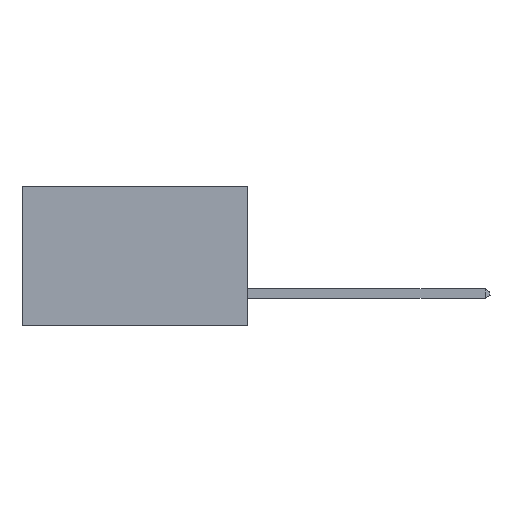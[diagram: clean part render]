
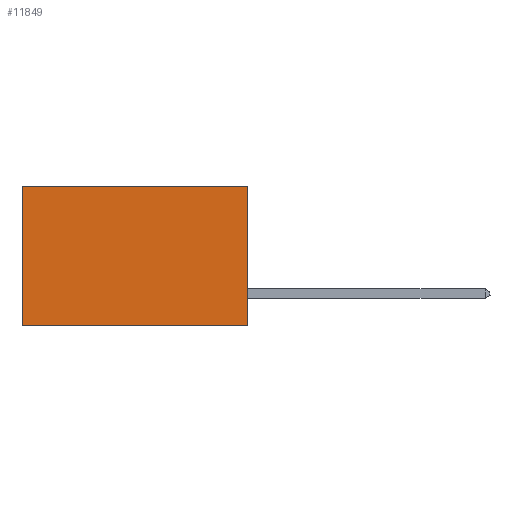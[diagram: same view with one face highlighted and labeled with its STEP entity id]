
A CAD part, left-side view. The second image highlights one B-rep face of the part: STEP entity #11849.
In plain terms, the highlighted planar face has unit normal (-1, 0, 0).
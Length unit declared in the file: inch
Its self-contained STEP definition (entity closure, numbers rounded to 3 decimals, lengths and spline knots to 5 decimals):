
#145 = EDGE_CURVE ( 'NONE', #5645, #9036, #12371, .T. ) ;
#515 = EDGE_CURVE ( 'NONE', #6734, #9036, #594, .T. ) ;
#594 = LINE ( 'NONE', #8430, #11598 ) ;
#1111 = EDGE_CURVE ( 'NONE', #6306, #6734, #10936, .T. ) ;
#1329 = DIRECTION ( 'NONE',  ( 0., 0., -1. ) ) ;
#1531 = AXIS2_PLACEMENT_3D ( 'NONE', #2247, #9335, #3285 ) ;
#1947 = CARTESIAN_POINT ( 'NONE',  ( 0.298, 0., 0. ) ) ;
#2247 = CARTESIAN_POINT ( 'NONE',  ( 0.298, 0., 0. ) ) ;
#3099 = CARTESIAN_POINT ( 'NONE',  ( 0.298, 0., 0. ) ) ;
#3152 = VECTOR ( 'NONE', #6441, 39.37008 ) ;
#3285 = DIRECTION ( 'NONE',  ( 0., 0., -1. ) ) ;
#3694 = ORIENTED_EDGE ( 'NONE', *, *, #1111, .T. ) ;
#4475 = DIRECTION ( 'NONE',  ( 0., 0., -1. ) ) ;
#4659 = LINE ( 'NONE', #9530, #10099 ) ;
#5645 = VERTEX_POINT ( 'NONE', #8923 ) ;
#5964 = VECTOR ( 'NONE', #10267, 39.37008 ) ;
#6306 = VERTEX_POINT ( 'NONE', #1947 ) ;
#6441 = DIRECTION ( 'NONE',  ( 0., 1., 0. ) ) ;
#6734 = VERTEX_POINT ( 'NONE', #7531 ) ;
#7344 = ORIENTED_EDGE ( 'NONE', *, *, #515, .T. ) ;
#7531 = CARTESIAN_POINT ( 'NONE',  ( 0.298, 0.6, 0. ) ) ;
#8396 = CARTESIAN_POINT ( 'NONE',  ( 0.298, 0., -0.37 ) ) ;
#8430 = CARTESIAN_POINT ( 'NONE',  ( 0.298, 0.6, 0. ) ) ;
#8923 = CARTESIAN_POINT ( 'NONE',  ( 0.298, 0., -0.37 ) ) ;
#9036 = VERTEX_POINT ( 'NONE', #10608 ) ;
#9072 = ORIENTED_EDGE ( 'NONE', *, *, #145, .F. ) ;
#9179 = ORIENTED_EDGE ( 'NONE', *, *, #9618, .F. ) ;
#9251 = PLANE ( 'NONE',  #1531 ) ;
#9335 = DIRECTION ( 'NONE',  ( 1., 0., 0. ) ) ;
#9530 = CARTESIAN_POINT ( 'NONE',  ( 0.298, 0., 0. ) ) ;
#9618 = EDGE_CURVE ( 'NONE', #6306, #5645, #4659, .T. ) ;
#10099 = VECTOR ( 'NONE', #4475, 39.37008 ) ;
#10267 = DIRECTION ( 'NONE',  ( 0., 1., 0. ) ) ;
#10608 = CARTESIAN_POINT ( 'NONE',  ( 0.298, 0.6, -0.37 ) ) ;
#10936 = LINE ( 'NONE', #3099, #5964 ) ;
#11598 = VECTOR ( 'NONE', #1329, 39.37008 ) ;
#11775 = EDGE_LOOP ( 'NONE', ( #7344, #9072, #9179, #3694 ) ) ;
#11849 = ADVANCED_FACE ( 'NONE', ( #12415 ), #9251, .F. ) ;
#12371 = LINE ( 'NONE', #8396, #3152 ) ;
#12415 = FACE_OUTER_BOUND ( 'NONE', #11775, .T. ) ;
